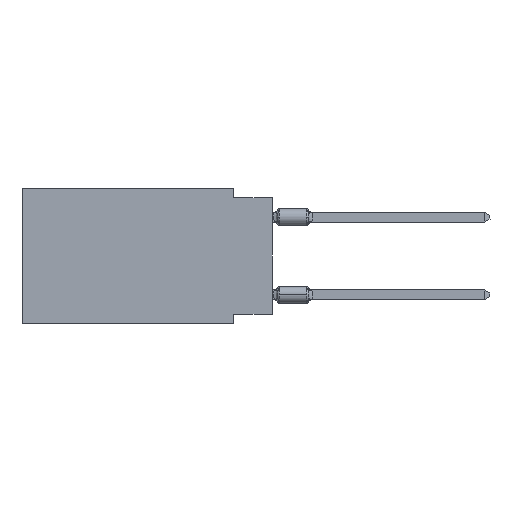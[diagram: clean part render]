
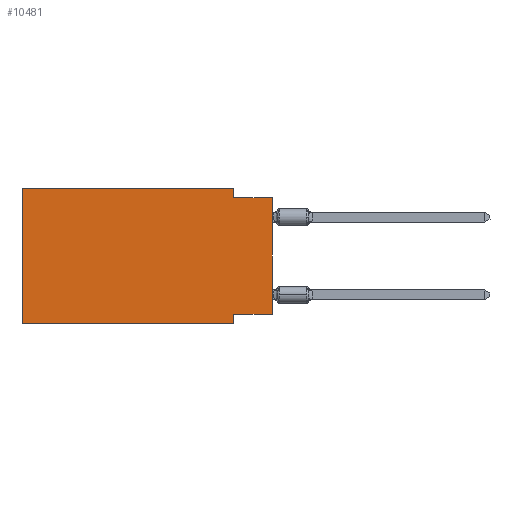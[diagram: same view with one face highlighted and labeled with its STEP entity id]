
A CAD part, left-side view. The second image highlights one B-rep face of the part: STEP entity #10481.
In plain terms, the highlighted planar face has unit normal (-1, 0, 0).
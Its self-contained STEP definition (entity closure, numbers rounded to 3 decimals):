
#99 = VECTOR ( 'NONE', #17488, 1000. ) ;
#100 = LINE ( 'NONE', #15596, #15317 ) ;
#285 = DIRECTION ( 'NONE',  ( 0., 1., 0. ) ) ;
#288 = EDGE_CURVE ( 'NONE', #4443, #15521, #1220, .T. ) ;
#317 = EDGE_CURVE ( 'NONE', #2551, #16509, #10216, .T. ) ;
#323 = DIRECTION ( 'NONE',  ( 1., 0., 0. ) ) ;
#352 = CARTESIAN_POINT ( 'NONE',  ( 0., 16.383, 0. ) ) ;
#748 = LINE ( 'NONE', #7708, #2708 ) ;
#1220 = LINE ( 'NONE', #11042, #11554 ) ;
#2018 = EDGE_CURVE ( 'NONE', #15521, #14050, #748, .T. ) ;
#2182 = EDGE_LOOP ( 'NONE', ( #12343, #4455, #8313, #11501, #8667, #16843, #14187, #11410 ) ) ;
#2489 = VECTOR ( 'NONE', #4525, 1000. ) ;
#2551 = VERTEX_POINT ( 'NONE', #10614 ) ;
#2561 = VECTOR ( 'NONE', #285, 1000. ) ;
#2708 = VECTOR ( 'NONE', #6336, 1000. ) ;
#3721 = LINE ( 'NONE', #10606, #99 ) ;
#3898 = CARTESIAN_POINT ( 'NONE',  ( 0., 2.54, -0.635 ) ) ;
#4443 = VERTEX_POINT ( 'NONE', #6368 ) ;
#4455 = ORIENTED_EDGE ( 'NONE', *, *, #5343, .F. ) ;
#4525 = DIRECTION ( 'NONE',  ( 0., 0., 1. ) ) ;
#5015 = VERTEX_POINT ( 'NONE', #7332 ) ;
#5343 = EDGE_CURVE ( 'NONE', #14050, #16509, #9898, .T. ) ;
#5617 = VECTOR ( 'NONE', #16482, 1000. ) ;
#5735 = DIRECTION ( 'NONE',  ( 0., 0., -1. ) ) ;
#6244 = EDGE_CURVE ( 'NONE', #2551, #14357, #14492, .T. ) ;
#6336 = DIRECTION ( 'NONE',  ( 0., 0., -1. ) ) ;
#6368 = CARTESIAN_POINT ( 'NONE',  ( 0., 16.383, 0. ) ) ;
#7332 = CARTESIAN_POINT ( 'NONE',  ( 0., 16.383, -8.89 ) ) ;
#7464 = CARTESIAN_POINT ( 'NONE',  ( 0., 0., 0. ) ) ;
#7708 = CARTESIAN_POINT ( 'NONE',  ( 0., 2.54, 0. ) ) ;
#7941 = CARTESIAN_POINT ( 'NONE',  ( 0., 2.54, -8.89 ) ) ;
#8313 = ORIENTED_EDGE ( 'NONE', *, *, #2018, .F. ) ;
#8667 = ORIENTED_EDGE ( 'NONE', *, *, #12497, .F. ) ;
#9898 = LINE ( 'NONE', #10883, #5617 ) ;
#10216 = LINE ( 'NONE', #7464, #2489 ) ;
#10251 = DIRECTION ( 'NONE',  ( 0., 0., 1. ) ) ;
#10481 = ADVANCED_FACE ( 'NONE', ( #12904 ), #15760, .F. ) ;
#10606 = CARTESIAN_POINT ( 'NONE',  ( 0., 2.54, -8.89 ) ) ;
#10614 = CARTESIAN_POINT ( 'NONE',  ( 0., 0., -8.255 ) ) ;
#10883 = CARTESIAN_POINT ( 'NONE',  ( 0., 0., -0.635 ) ) ;
#11013 = DIRECTION ( 'NONE',  ( 0., -1., 0. ) ) ;
#11042 = CARTESIAN_POINT ( 'NONE',  ( 0., 16.383, 0. ) ) ;
#11410 = ORIENTED_EDGE ( 'NONE', *, *, #6244, .F. ) ;
#11501 = ORIENTED_EDGE ( 'NONE', *, *, #288, .F. ) ;
#11554 = VECTOR ( 'NONE', #16629, 1000. ) ;
#12343 = ORIENTED_EDGE ( 'NONE', *, *, #317, .T. ) ;
#12497 = EDGE_CURVE ( 'NONE', #5015, #4443, #17129, .T. ) ;
#12723 = VERTEX_POINT ( 'NONE', #7941 ) ;
#12811 = CARTESIAN_POINT ( 'NONE',  ( 0., 16.383, 0. ) ) ;
#12904 = FACE_OUTER_BOUND ( 'NONE', #2182, .T. ) ;
#12909 = CARTESIAN_POINT ( 'NONE',  ( 0., 2.54, 0. ) ) ;
#13149 = EDGE_CURVE ( 'NONE', #5015, #12723, #100, .T. ) ;
#13932 = EDGE_CURVE ( 'NONE', #14357, #12723, #3721, .T. ) ;
#14050 = VERTEX_POINT ( 'NONE', #3898 ) ;
#14147 = AXIS2_PLACEMENT_3D ( 'NONE', #352, #323, #5735 ) ;
#14187 = ORIENTED_EDGE ( 'NONE', *, *, #13932, .F. ) ;
#14313 = CARTESIAN_POINT ( 'NONE',  ( 0., 0., -8.255 ) ) ;
#14357 = VERTEX_POINT ( 'NONE', #16351 ) ;
#14492 = LINE ( 'NONE', #14313, #2561 ) ;
#14910 = VECTOR ( 'NONE', #10251, 1000. ) ;
#15317 = VECTOR ( 'NONE', #11013, 1000. ) ;
#15521 = VERTEX_POINT ( 'NONE', #12909 ) ;
#15596 = CARTESIAN_POINT ( 'NONE',  ( 0., 16.383, -8.89 ) ) ;
#15760 = PLANE ( 'NONE',  #14147 ) ;
#16351 = CARTESIAN_POINT ( 'NONE',  ( 0., 2.54, -8.255 ) ) ;
#16482 = DIRECTION ( 'NONE',  ( 0., -1., 0. ) ) ;
#16509 = VERTEX_POINT ( 'NONE', #16768 ) ;
#16629 = DIRECTION ( 'NONE',  ( 0., -1., 0. ) ) ;
#16768 = CARTESIAN_POINT ( 'NONE',  ( 0., 0., -0.635 ) ) ;
#16843 = ORIENTED_EDGE ( 'NONE', *, *, #13149, .T. ) ;
#17129 = LINE ( 'NONE', #12811, #14910 ) ;
#17488 = DIRECTION ( 'NONE',  ( 0., 0., -1. ) ) ;
